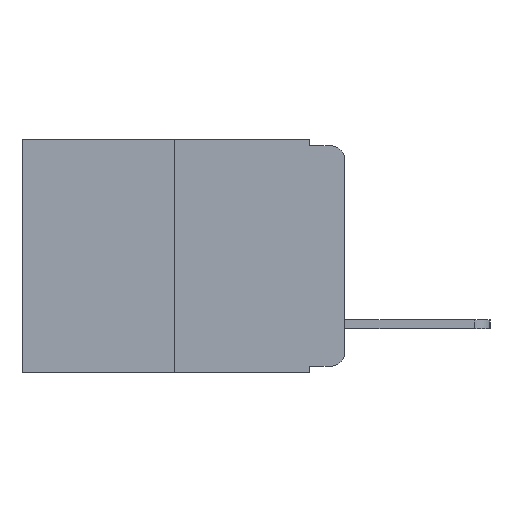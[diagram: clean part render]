
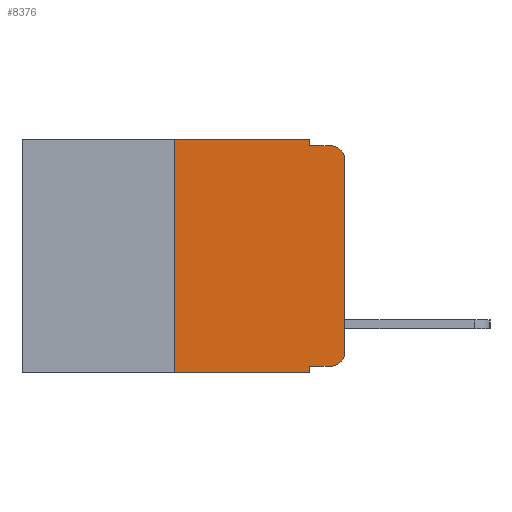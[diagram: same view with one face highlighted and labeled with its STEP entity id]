
A CAD part, left-side view. The second image highlights one B-rep face of the part: STEP entity #8376.
In plain terms, the highlighted planar face has unit normal (-1, 0, 0).
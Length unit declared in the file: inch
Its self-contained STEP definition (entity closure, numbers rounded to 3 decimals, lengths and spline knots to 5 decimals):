
#73 = LINE ( 'NONE', #17119, #18949 ) ;
#132 = VERTEX_POINT ( 'NONE', #9952 ) ;
#1407 = CARTESIAN_POINT ( 'NONE',  ( 0., 0., -0.313 ) ) ;
#1488 = EDGE_CURVE ( 'NONE', #5946, #6559, #11905, .T. ) ;
#1653 = LINE ( 'NONE', #12938, #4774 ) ;
#1854 = LINE ( 'NONE', #3904, #12945 ) ;
#2294 = CARTESIAN_POINT ( 'NONE',  ( 0., 0.473, 0. ) ) ;
#2445 = ORIENTED_EDGE ( 'NONE', *, *, #17046, .F. ) ;
#2578 = CIRCLE ( 'NONE', #16048, 0.02 ) ;
#3105 = LINE ( 'NONE', #16810, #10703 ) ;
#3569 = EDGE_CURVE ( 'NONE', #7585, #9149, #2578, .T. ) ;
#3593 = LINE ( 'NONE', #2294, #18854 ) ;
#3693 = DIRECTION ( 'NONE',  ( 0., -1., 0. ) ) ;
#3904 = CARTESIAN_POINT ( 'NONE',  ( 0., 0.051, 0. ) ) ;
#3918 = EDGE_CURVE ( 'NONE', #12364, #5946, #15732, .T. ) ;
#4774 = VECTOR ( 'NONE', #5493, 39.37008 ) ;
#4868 = ORIENTED_EDGE ( 'NONE', *, *, #18986, .F. ) ;
#4894 = DIRECTION ( 'NONE',  ( 0., -1., 0. ) ) ;
#5461 = FACE_OUTER_BOUND ( 'NONE', #10306, .T. ) ;
#5493 = DIRECTION ( 'NONE',  ( 0., 0., 1. ) ) ;
#5655 = DIRECTION ( 'NONE',  ( 0., 0., -1. ) ) ;
#5842 = ORIENTED_EDGE ( 'NONE', *, *, #8358, .F. ) ;
#5946 = VERTEX_POINT ( 'NONE', #7519 ) ;
#6274 = EDGE_CURVE ( 'NONE', #12471, #132, #73, .T. ) ;
#6476 = EDGE_CURVE ( 'NONE', #6559, #7585, #18714, .T. ) ;
#6559 = VERTEX_POINT ( 'NONE', #1407 ) ;
#7040 = VECTOR ( 'NONE', #18989, 39.37008 ) ;
#7223 = CARTESIAN_POINT ( 'NONE',  ( 0., 0.051, 0. ) ) ;
#7519 = CARTESIAN_POINT ( 'NONE',  ( 0., 0.02, -0.333 ) ) ;
#7585 = VERTEX_POINT ( 'NONE', #14666 ) ;
#7754 = EDGE_CURVE ( 'NONE', #12471, #19258, #1653, .T. ) ;
#8357 = VERTEX_POINT ( 'NONE', #8409 ) ;
#8358 = EDGE_CURVE ( 'NONE', #12364, #132, #1854, .T. ) ;
#8376 = ADVANCED_FACE ( 'NONE', ( #5461 ), #15937, .F. ) ;
#8409 = CARTESIAN_POINT ( 'NONE',  ( 0., 0.051, -0.01 ) ) ;
#8432 = CARTESIAN_POINT ( 'NONE',  ( 0., 0.051, -0.01 ) ) ;
#9054 = CARTESIAN_POINT ( 'NONE',  ( 0., 0.02, -0.03 ) ) ;
#9149 = VERTEX_POINT ( 'NONE', #13282 ) ;
#9952 = CARTESIAN_POINT ( 'NONE',  ( 0., 0.051, -0.343 ) ) ;
#9966 = DIRECTION ( 'NONE',  ( 0., -1., 0. ) ) ;
#10072 = DIRECTION ( 'NONE',  ( 0., 0., -1. ) ) ;
#10306 = EDGE_LOOP ( 'NONE', ( #17397, #13987, #2445, #10979, #4868, #12837, #13302, #5842, #14511, #10498 ) ) ;
#10334 = CARTESIAN_POINT ( 'NONE',  ( 0., 0.051, -0.333 ) ) ;
#10498 = ORIENTED_EDGE ( 'NONE', *, *, #1488, .T. ) ;
#10703 = VECTOR ( 'NONE', #18230, 39.37008 ) ;
#10722 = AXIS2_PLACEMENT_3D ( 'NONE', #12868, #12975, #13085 ) ;
#10979 = ORIENTED_EDGE ( 'NONE', *, *, #13512, .F. ) ;
#11433 = DIRECTION ( 'NONE',  ( 0., -1., 0. ) ) ;
#11831 = VECTOR ( 'NONE', #4894, 39.37008 ) ;
#11905 = CIRCLE ( 'NONE', #10722, 0.02 ) ;
#12021 = CARTESIAN_POINT ( 'NONE',  ( 0., 0.051, -0.333 ) ) ;
#12364 = VERTEX_POINT ( 'NONE', #10334 ) ;
#12471 = VERTEX_POINT ( 'NONE', #13564 ) ;
#12837 = ORIENTED_EDGE ( 'NONE', *, *, #7754, .F. ) ;
#12868 = CARTESIAN_POINT ( 'NONE',  ( 0., 0.02, -0.313 ) ) ;
#12938 = CARTESIAN_POINT ( 'NONE',  ( 0., 0.25, 0. ) ) ;
#12945 = VECTOR ( 'NONE', #18695, 39.37008 ) ;
#12975 = DIRECTION ( 'NONE',  ( -1., 0., 0. ) ) ;
#13085 = DIRECTION ( 'NONE',  ( 0., 0., -1. ) ) ;
#13282 = CARTESIAN_POINT ( 'NONE',  ( 0., 0.02, -0.01 ) ) ;
#13302 = ORIENTED_EDGE ( 'NONE', *, *, #6274, .T. ) ;
#13512 = EDGE_CURVE ( 'NONE', #14304, #8357, #3105, .T. ) ;
#13564 = CARTESIAN_POINT ( 'NONE',  ( 0., 0.25, -0.343 ) ) ;
#13987 = ORIENTED_EDGE ( 'NONE', *, *, #3569, .T. ) ;
#14304 = VERTEX_POINT ( 'NONE', #7223 ) ;
#14511 = ORIENTED_EDGE ( 'NONE', *, *, #3918, .T. ) ;
#14565 = DIRECTION ( 'NONE',  ( -1., 0., 0. ) ) ;
#14666 = CARTESIAN_POINT ( 'NONE',  ( 0., 0., -0.03 ) ) ;
#14921 = AXIS2_PLACEMENT_3D ( 'NONE', #17380, #18763, #10072 ) ;
#15732 = LINE ( 'NONE', #12021, #11831 ) ;
#15937 = PLANE ( 'NONE',  #14921 ) ;
#16048 = AXIS2_PLACEMENT_3D ( 'NONE', #9054, #14565, #5655 ) ;
#16810 = CARTESIAN_POINT ( 'NONE',  ( 0., 0.051, 0. ) ) ;
#17046 = EDGE_CURVE ( 'NONE', #8357, #9149, #18308, .T. ) ;
#17119 = CARTESIAN_POINT ( 'NONE',  ( 0., 0.473, -0.343 ) ) ;
#17380 = CARTESIAN_POINT ( 'NONE',  ( 0., 0.473, 0. ) ) ;
#17397 = ORIENTED_EDGE ( 'NONE', *, *, #6476, .T. ) ;
#17623 = CARTESIAN_POINT ( 'NONE',  ( 0., 0., 0. ) ) ;
#17905 = VECTOR ( 'NONE', #9966, 39.37008 ) ;
#18230 = DIRECTION ( 'NONE',  ( 0., 0., -1. ) ) ;
#18308 = LINE ( 'NONE', #8432, #17905 ) ;
#18695 = DIRECTION ( 'NONE',  ( 0., 0., -1. ) ) ;
#18714 = LINE ( 'NONE', #17623, #7040 ) ;
#18763 = DIRECTION ( 'NONE',  ( 1., 0., 0. ) ) ;
#18854 = VECTOR ( 'NONE', #11433, 39.37008 ) ;
#18949 = VECTOR ( 'NONE', #3693, 39.37008 ) ;
#18986 = EDGE_CURVE ( 'NONE', #19258, #14304, #3593, .T. ) ;
#18989 = DIRECTION ( 'NONE',  ( 0., 0., 1. ) ) ;
#19234 = CARTESIAN_POINT ( 'NONE',  ( 0., 0.25, 0. ) ) ;
#19258 = VERTEX_POINT ( 'NONE', #19234 ) ;
